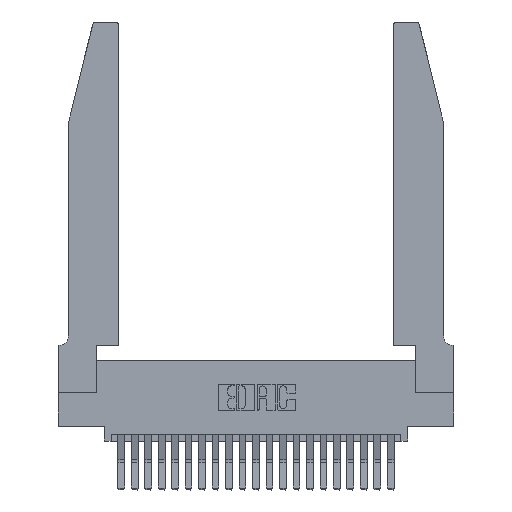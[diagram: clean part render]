
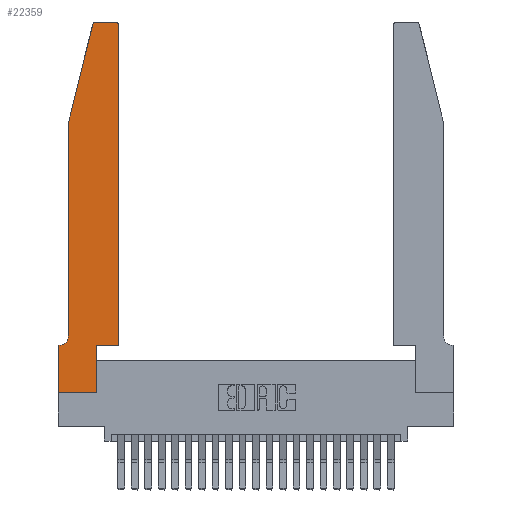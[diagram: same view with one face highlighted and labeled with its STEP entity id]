
A CAD part, top view. The second image highlights one B-rep face of the part: STEP entity #22359.
In plain terms, the highlighted planar face has unit normal (0, 0, 1).
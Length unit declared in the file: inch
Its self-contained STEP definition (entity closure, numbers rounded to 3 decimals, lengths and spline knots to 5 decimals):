
#497 = VERTEX_POINT ( 'NONE', #7011 ) ;
#538 = EDGE_CURVE ( 'NONE', #578, #497, #23972, .T. ) ;
#578 = VERTEX_POINT ( 'NONE', #7302 ) ;
#795 = DIRECTION ( 'NONE',  ( 1., 0., 0. ) ) ;
#1445 = DIRECTION ( 'NONE',  ( 1., 0., 0. ) ) ;
#2007 = CARTESIAN_POINT ( 'NONE',  ( 0.0055, 0.42, 0.37 ) ) ;
#2026 = ORIENTED_EDGE ( 'NONE', *, *, #13921, .T. ) ;
#2344 = LINE ( 'NONE', #21454, #2833 ) ;
#2522 = EDGE_CURVE ( 'NONE', #11344, #9320, #11052, .T. ) ;
#2639 = CARTESIAN_POINT ( 'NONE',  ( 0.2865, 0.35, 0.37 ) ) ;
#2833 = VECTOR ( 'NONE', #5910, 39.37008 ) ;
#3472 = CARTESIAN_POINT ( 'NONE',  ( 0.4505, 0.35, 0.37 ) ) ;
#3709 = AXIS2_PLACEMENT_3D ( 'NONE', #23851, #12627, #12468 ) ;
#3776 = ORIENTED_EDGE ( 'NONE', *, *, #4635, .T. ) ;
#3878 = VECTOR ( 'NONE', #13748, 39.37008 ) ;
#3888 = DIRECTION ( 'NONE',  ( -1., 0., 0. ) ) ;
#4077 = LINE ( 'NONE', #16304, #14673 ) ;
#4127 = VERTEX_POINT ( 'NONE', #7839 ) ;
#4376 = VERTEX_POINT ( 'NONE', #12095 ) ;
#4497 = CARTESIAN_POINT ( 'NONE',  ( 0.4505, 0.35, 0.37 ) ) ;
#4635 = EDGE_CURVE ( 'NONE', #12520, #11344, #21455, .T. ) ;
#4953 = ORIENTED_EDGE ( 'NONE', *, *, #6953, .T. ) ;
#4970 = CARTESIAN_POINT ( 'NONE',  ( 0.0755, 0.42, 0.37 ) ) ;
#5059 = CARTESIAN_POINT ( 'NONE',  ( 0., 0.35, 0.37 ) ) ;
#5910 = DIRECTION ( 'NONE',  ( 0., 1., 0. ) ) ;
#5955 = DIRECTION ( 'NONE',  ( 0., 0., -1. ) ) ;
#6073 = CIRCLE ( 'NONE', #18460, 0.03 ) ;
#6650 = ORIENTED_EDGE ( 'NONE', *, *, #2522, .T. ) ;
#6864 = ORIENTED_EDGE ( 'NONE', *, *, #21320, .T. ) ;
#6880 = ORIENTED_EDGE ( 'NONE', *, *, #12188, .T. ) ;
#6953 = EDGE_CURVE ( 'NONE', #22358, #4376, #18166, .T. ) ;
#6987 = DIRECTION ( 'NONE',  ( 1., 0., 0. ) ) ;
#7011 = CARTESIAN_POINT ( 'NONE',  ( 0.2865, 0., 0.37 ) ) ;
#7302 = CARTESIAN_POINT ( 'NONE',  ( 0., 0., 0.37 ) ) ;
#7304 = EDGE_CURVE ( 'NONE', #4127, #578, #19907, .T. ) ;
#7430 = CARTESIAN_POINT ( 'NONE',  ( 0.0755, 2., 0.37 ) ) ;
#7839 = CARTESIAN_POINT ( 'NONE',  ( 0., 0.35, 0.37 ) ) ;
#8360 = CARTESIAN_POINT ( 'NONE',  ( 0.284, 2.75, 0.37 ) ) ;
#8481 = ORIENTED_EDGE ( 'NONE', *, *, #17805, .T. ) ;
#8797 = VERTEX_POINT ( 'NONE', #3472 ) ;
#9320 = VERTEX_POINT ( 'NONE', #14374 ) ;
#9952 = VECTOR ( 'NONE', #23375, 39.37008 ) ;
#10558 = CARTESIAN_POINT ( 'NONE',  ( 0.4505, 2.72, 0.37 ) ) ;
#10887 = VERTEX_POINT ( 'NONE', #23549 ) ;
#11052 = CIRCLE ( 'NONE', #3709, 0.03 ) ;
#11122 = DIRECTION ( 'NONE',  ( -1., 0., 0. ) ) ;
#11344 = VERTEX_POINT ( 'NONE', #8360 ) ;
#11433 = EDGE_LOOP ( 'NONE', ( #3776, #6650, #17647, #23842, #4953, #8481, #21433, #13379, #17274, #6864, #6880, #2026 ) ) ;
#11750 = EDGE_CURVE ( 'NONE', #11773, #22358, #22018, .T. ) ;
#11773 = VERTEX_POINT ( 'NONE', #23006 ) ;
#12095 = CARTESIAN_POINT ( 'NONE',  ( 0.0055, 0.35, 0.37 ) ) ;
#12188 = EDGE_CURVE ( 'NONE', #8797, #17581, #2344, .T. ) ;
#12468 = DIRECTION ( 'NONE',  ( 1., 0., 0. ) ) ;
#12520 = VERTEX_POINT ( 'NONE', #24290 ) ;
#12627 = DIRECTION ( 'NONE',  ( 0., 0., 1. ) ) ;
#12752 = DIRECTION ( 'NONE',  ( 0., 0., 1. ) ) ;
#13197 = DIRECTION ( 'NONE',  ( 0., -1., 0. ) ) ;
#13379 = ORIENTED_EDGE ( 'NONE', *, *, #538, .T. ) ;
#13517 = AXIS2_PLACEMENT_3D ( 'NONE', #5059, #22038, #1445 ) ;
#13748 = DIRECTION ( 'NONE',  ( -1., 0., 0. ) ) ;
#13921 = EDGE_CURVE ( 'NONE', #17581, #12520, #6073, .T. ) ;
#14374 = CARTESIAN_POINT ( 'NONE',  ( 0.25487, 2.72718, 0.37 ) ) ;
#14673 = VECTOR ( 'NONE', #11122, 39.37008 ) ;
#14962 = VECTOR ( 'NONE', #18379, 39.37008 ) ;
#15252 = AXIS2_PLACEMENT_3D ( 'NONE', #2007, #5955, #3888 ) ;
#15326 = LINE ( 'NONE', #4497, #23830 ) ;
#16304 = CARTESIAN_POINT ( 'NONE',  ( 0.0755, 0.35, 0.37 ) ) ;
#16598 = CARTESIAN_POINT ( 'NONE',  ( 0.4205, 2.72, 0.37 ) ) ;
#17274 = ORIENTED_EDGE ( 'NONE', *, *, #23249, .T. ) ;
#17565 = DIRECTION ( 'NONE',  ( -0.239, -0.971, 0. ) ) ;
#17581 = VERTEX_POINT ( 'NONE', #10558 ) ;
#17647 = ORIENTED_EDGE ( 'NONE', *, *, #18697, .T. ) ;
#17805 = EDGE_CURVE ( 'NONE', #4376, #4127, #4077, .T. ) ;
#18166 = CIRCLE ( 'NONE', #15252, 0.07 ) ;
#18211 = CARTESIAN_POINT ( 'NONE',  ( 0., 0., 0.37 ) ) ;
#18379 = DIRECTION ( 'NONE',  ( 0., -1., 0. ) ) ;
#18385 = VECTOR ( 'NONE', #6987, 39.37008 ) ;
#18460 = AXIS2_PLACEMENT_3D ( 'NONE', #16598, #12752, #22479 ) ;
#18697 = EDGE_CURVE ( 'NONE', #9320, #11773, #22514, .T. ) ;
#19161 = CARTESIAN_POINT ( 'NONE',  ( 0.0755, 2., 0.37 ) ) ;
#19286 = CARTESIAN_POINT ( 'NONE',  ( 0., 0., 0.37 ) ) ;
#19307 = LINE ( 'NONE', #2639, #9952 ) ;
#19848 = VECTOR ( 'NONE', #17565, 39.37008 ) ;
#19907 = LINE ( 'NONE', #18211, #14962 ) ;
#21320 = EDGE_CURVE ( 'NONE', #10887, #8797, #15326, .T. ) ;
#21433 = ORIENTED_EDGE ( 'NONE', *, *, #7304, .T. ) ;
#21454 = CARTESIAN_POINT ( 'NONE',  ( 0.4505, 0.35, 0.37 ) ) ;
#21455 = LINE ( 'NONE', #22692, #3878 ) ;
#21693 = FACE_OUTER_BOUND ( 'NONE', #11433, .T. ) ;
#22018 = LINE ( 'NONE', #7430, #22877 ) ;
#22038 = DIRECTION ( 'NONE',  ( 0., 0., 1. ) ) ;
#22358 = VERTEX_POINT ( 'NONE', #4970 ) ;
#22359 = ADVANCED_FACE ( 'NONE', ( #21693 ), #23839, .T. ) ;
#22479 = DIRECTION ( 'NONE',  ( 1., 0., 0. ) ) ;
#22514 = LINE ( 'NONE', #19161, #19848 ) ;
#22692 = CARTESIAN_POINT ( 'NONE',  ( 0.2605, 2.75, 0.37 ) ) ;
#22877 = VECTOR ( 'NONE', #13197, 39.37008 ) ;
#23006 = CARTESIAN_POINT ( 'NONE',  ( 0.0755, 2., 0.37 ) ) ;
#23249 = EDGE_CURVE ( 'NONE', #497, #10887, #19307, .T. ) ;
#23375 = DIRECTION ( 'NONE',  ( 0., 1., 0. ) ) ;
#23549 = CARTESIAN_POINT ( 'NONE',  ( 0.2865, 0.35, 0.37 ) ) ;
#23830 = VECTOR ( 'NONE', #795, 39.37008 ) ;
#23839 = PLANE ( 'NONE',  #13517 ) ;
#23842 = ORIENTED_EDGE ( 'NONE', *, *, #11750, .T. ) ;
#23851 = CARTESIAN_POINT ( 'NONE',  ( 0.284, 2.72, 0.37 ) ) ;
#23972 = LINE ( 'NONE', #19286, #18385 ) ;
#24290 = CARTESIAN_POINT ( 'NONE',  ( 0.4205, 2.75, 0.37 ) ) ;
